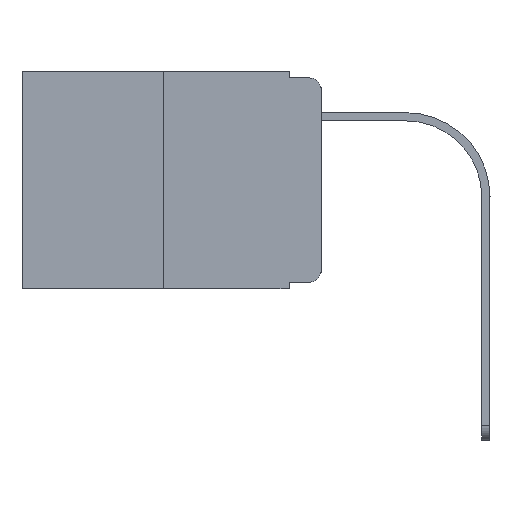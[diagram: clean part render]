
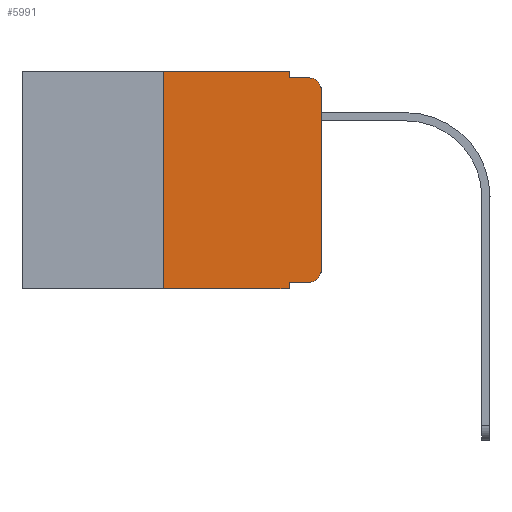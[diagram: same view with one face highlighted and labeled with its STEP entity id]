
A CAD part, left-side view. The second image highlights one B-rep face of the part: STEP entity #5991.
In plain terms, the highlighted planar face has unit normal (-1, 0, 0).
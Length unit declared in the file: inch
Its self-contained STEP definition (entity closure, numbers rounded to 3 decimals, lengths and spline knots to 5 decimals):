
#2 = AXIS2_PLACEMENT_3D ( 'NONE', #3297, #8537, #7314 ) ;
#279 = CARTESIAN_POINT ( 'NONE',  ( 0., 0.051, -0.333 ) ) ;
#286 = VERTEX_POINT ( 'NONE', #6278 ) ;
#442 = LINE ( 'NONE', #6898, #5333 ) ;
#477 = DIRECTION ( 'NONE',  ( 0., -1., 0. ) ) ;
#838 = CARTESIAN_POINT ( 'NONE',  ( 0., 0.473, 0. ) ) ;
#1096 = CARTESIAN_POINT ( 'NONE',  ( 0., 0., 0. ) ) ;
#1488 = AXIS2_PLACEMENT_3D ( 'NONE', #838, #12253, #4954 ) ;
#1503 = AXIS2_PLACEMENT_3D ( 'NONE', #3586, #8761, #5655 ) ;
#1546 = VERTEX_POINT ( 'NONE', #7516 ) ;
#1730 = VECTOR ( 'NONE', #11743, 39.37008 ) ;
#1744 = ORIENTED_EDGE ( 'NONE', *, *, #7100, .T. ) ;
#1766 = EDGE_LOOP ( 'NONE', ( #7168, #1918, #8518, #12464, #4400, #7790, #1744, #10025, #8587, #13290 ) ) ;
#1918 = ORIENTED_EDGE ( 'NONE', *, *, #4988, .T. ) ;
#2080 = DIRECTION ( 'NONE',  ( 0., 0., 1. ) ) ;
#2442 = CARTESIAN_POINT ( 'NONE',  ( 0., 0.473, -0.343 ) ) ;
#2598 = LINE ( 'NONE', #3685, #1730 ) ;
#3004 = VERTEX_POINT ( 'NONE', #8459 ) ;
#3297 = CARTESIAN_POINT ( 'NONE',  ( 0., 0.02, -0.313 ) ) ;
#3414 = CARTESIAN_POINT ( 'NONE',  ( 0., 0.051, -0.01 ) ) ;
#3586 = CARTESIAN_POINT ( 'NONE',  ( 0., 0.02, -0.03 ) ) ;
#3685 = CARTESIAN_POINT ( 'NONE',  ( 0., 0.051, 0. ) ) ;
#3993 = EDGE_CURVE ( 'NONE', #286, #3004, #442, .T. ) ;
#4016 = FACE_OUTER_BOUND ( 'NONE', #1766, .T. ) ;
#4048 = LINE ( 'NONE', #7074, #9376 ) ;
#4400 = ORIENTED_EDGE ( 'NONE', *, *, #12701, .F. ) ;
#4618 = EDGE_CURVE ( 'NONE', #9826, #9738, #6422, .T. ) ;
#4666 = VERTEX_POINT ( 'NONE', #10038 ) ;
#4954 = DIRECTION ( 'NONE',  ( 0., 0., -1. ) ) ;
#4967 = CIRCLE ( 'NONE', #2, 0.02 ) ;
#4988 = EDGE_CURVE ( 'NONE', #10928, #5117, #12715, .T. ) ;
#5117 = VERTEX_POINT ( 'NONE', #5177 ) ;
#5177 = CARTESIAN_POINT ( 'NONE',  ( 0., 0.02, -0.01 ) ) ;
#5304 = CARTESIAN_POINT ( 'NONE',  ( 0., 0.473, 0. ) ) ;
#5333 = VECTOR ( 'NONE', #9944, 39.37008 ) ;
#5655 = DIRECTION ( 'NONE',  ( 0., 0., -1. ) ) ;
#5991 = ADVANCED_FACE ( 'NONE', ( #4016 ), #10008, .F. ) ;
#6278 = CARTESIAN_POINT ( 'NONE',  ( 0., 0.051, 0. ) ) ;
#6422 = LINE ( 'NONE', #279, #9247 ) ;
#6438 = CARTESIAN_POINT ( 'NONE',  ( 0., 0., -0.313 ) ) ;
#6503 = EDGE_CURVE ( 'NONE', #13173, #10928, #10342, .T. ) ;
#6561 = DIRECTION ( 'NONE',  ( 0., -1., 0. ) ) ;
#6564 = VECTOR ( 'NONE', #7488, 39.37008 ) ;
#6898 = CARTESIAN_POINT ( 'NONE',  ( 0., 0.051, 0. ) ) ;
#7074 = CARTESIAN_POINT ( 'NONE',  ( 0., 0.25, 0. ) ) ;
#7100 = EDGE_CURVE ( 'NONE', #1546, #11311, #11706, .T. ) ;
#7168 = ORIENTED_EDGE ( 'NONE', *, *, #6503, .T. ) ;
#7186 = DIRECTION ( 'NONE',  ( 0., -1., 0. ) ) ;
#7314 = DIRECTION ( 'NONE',  ( 0., 0., -1. ) ) ;
#7488 = DIRECTION ( 'NONE',  ( 0., -1., 0. ) ) ;
#7516 = CARTESIAN_POINT ( 'NONE',  ( 0., 0.25, -0.343 ) ) ;
#7790 = ORIENTED_EDGE ( 'NONE', *, *, #13278, .F. ) ;
#7823 = EDGE_CURVE ( 'NONE', #9738, #13173, #4967, .T. ) ;
#7957 = EDGE_CURVE ( 'NONE', #9826, #11311, #2598, .T. ) ;
#8043 = VECTOR ( 'NONE', #7186, 39.37008 ) ;
#8164 = VECTOR ( 'NONE', #6561, 39.37008 ) ;
#8194 = CARTESIAN_POINT ( 'NONE',  ( 0., 0.051, -0.343 ) ) ;
#8459 = CARTESIAN_POINT ( 'NONE',  ( 0., 0.051, -0.01 ) ) ;
#8518 = ORIENTED_EDGE ( 'NONE', *, *, #13128, .F. ) ;
#8537 = DIRECTION ( 'NONE',  ( -1., 0., 0. ) ) ;
#8581 = LINE ( 'NONE', #3414, #6564 ) ;
#8587 = ORIENTED_EDGE ( 'NONE', *, *, #4618, .T. ) ;
#8761 = DIRECTION ( 'NONE',  ( -1., 0., 0. ) ) ;
#9230 = LINE ( 'NONE', #5304, #8043 ) ;
#9247 = VECTOR ( 'NONE', #477, 39.37008 ) ;
#9337 = DIRECTION ( 'NONE',  ( 0., 0., 1. ) ) ;
#9376 = VECTOR ( 'NONE', #2080, 39.37008 ) ;
#9525 = CARTESIAN_POINT ( 'NONE',  ( 0., 0.051, -0.333 ) ) ;
#9690 = VECTOR ( 'NONE', #9337, 39.37008 ) ;
#9738 = VERTEX_POINT ( 'NONE', #11615 ) ;
#9826 = VERTEX_POINT ( 'NONE', #9525 ) ;
#9944 = DIRECTION ( 'NONE',  ( 0., 0., -1. ) ) ;
#10008 = PLANE ( 'NONE',  #1488 ) ;
#10025 = ORIENTED_EDGE ( 'NONE', *, *, #7957, .F. ) ;
#10038 = CARTESIAN_POINT ( 'NONE',  ( 0., 0.25, 0. ) ) ;
#10342 = LINE ( 'NONE', #1096, #9690 ) ;
#10928 = VERTEX_POINT ( 'NONE', #11349 ) ;
#11311 = VERTEX_POINT ( 'NONE', #8194 ) ;
#11349 = CARTESIAN_POINT ( 'NONE',  ( 0., 0., -0.03 ) ) ;
#11615 = CARTESIAN_POINT ( 'NONE',  ( 0., 0.02, -0.333 ) ) ;
#11706 = LINE ( 'NONE', #2442, #8164 ) ;
#11743 = DIRECTION ( 'NONE',  ( 0., 0., -1. ) ) ;
#12253 = DIRECTION ( 'NONE',  ( 1., 0., 0. ) ) ;
#12464 = ORIENTED_EDGE ( 'NONE', *, *, #3993, .F. ) ;
#12701 = EDGE_CURVE ( 'NONE', #4666, #286, #9230, .T. ) ;
#12715 = CIRCLE ( 'NONE', #1503, 0.02 ) ;
#13128 = EDGE_CURVE ( 'NONE', #3004, #5117, #8581, .T. ) ;
#13173 = VERTEX_POINT ( 'NONE', #6438 ) ;
#13278 = EDGE_CURVE ( 'NONE', #1546, #4666, #4048, .T. ) ;
#13290 = ORIENTED_EDGE ( 'NONE', *, *, #7823, .T. ) ;
